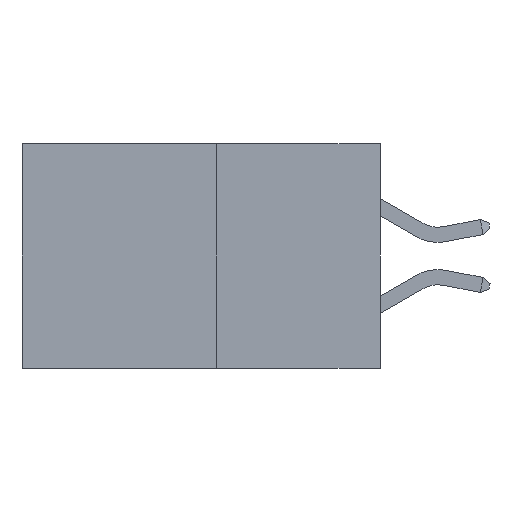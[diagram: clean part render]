
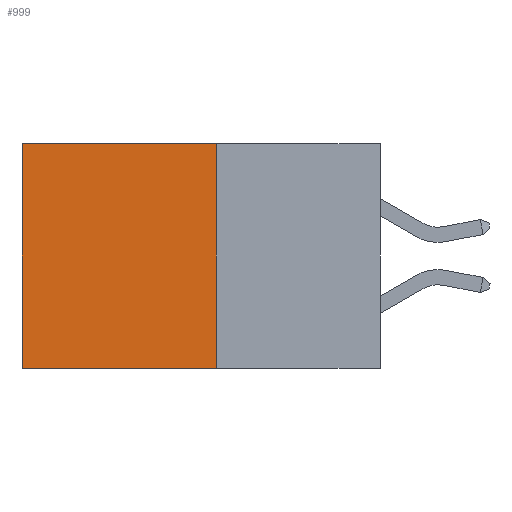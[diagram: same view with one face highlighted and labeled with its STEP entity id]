
A CAD part, left-side view. The second image highlights one B-rep face of the part: STEP entity #999.
In plain terms, the highlighted planar face has unit normal (-1, 0, 0).
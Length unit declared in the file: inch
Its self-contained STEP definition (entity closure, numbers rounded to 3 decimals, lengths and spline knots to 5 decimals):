
#92 = VERTEX_POINT ( 'NONE', #8112 ) ;
#236 = LINE ( 'NONE', #5766, #2025 ) ;
#418 = LINE ( 'NONE', #3237, #6210 ) ;
#638 = ORIENTED_EDGE ( 'NONE', *, *, #937, .F. ) ;
#935 = VECTOR ( 'NONE', #5083, 39.37008 ) ;
#937 = EDGE_CURVE ( 'NONE', #7355, #5221, #236, .T. ) ;
#999 = ADVANCED_FACE ( 'NONE', ( #5289 ), #2363, .F. ) ;
#2025 = VECTOR ( 'NONE', #2030, 39.37008 ) ;
#2030 = DIRECTION ( 'NONE',  ( 0., 0., -1. ) ) ;
#2363 = PLANE ( 'NONE',  #3022 ) ;
#2632 = ORIENTED_EDGE ( 'NONE', *, *, #5029, .T. ) ;
#3022 = AXIS2_PLACEMENT_3D ( 'NONE', #3222, #3078, #7476 ) ;
#3078 = DIRECTION ( 'NONE',  ( 1., 0., 0. ) ) ;
#3222 = CARTESIAN_POINT ( 'NONE',  ( 0.277, 0.27, -0.37 ) ) ;
#3237 = CARTESIAN_POINT ( 'NONE',  ( 0.277, 0.27, -0.37 ) ) ;
#3325 = EDGE_LOOP ( 'NONE', ( #6174, #8349, #638, #2632 ) ) ;
#3417 = EDGE_CURVE ( 'NONE', #5576, #92, #6691, .T. ) ;
#3563 = CARTESIAN_POINT ( 'NONE',  ( 0.277, 0.59, -0.37 ) ) ;
#3628 = CARTESIAN_POINT ( 'NONE',  ( 0.277, 0.27, -0.37 ) ) ;
#3979 = DIRECTION ( 'NONE',  ( 0., 1., 0. ) ) ;
#4792 = CARTESIAN_POINT ( 'NONE',  ( 0.277, 0.59, 0. ) ) ;
#5029 = EDGE_CURVE ( 'NONE', #7355, #5576, #6003, .T. ) ;
#5077 = CARTESIAN_POINT ( 'NONE',  ( 0.277, 0.27, 0. ) ) ;
#5083 = DIRECTION ( 'NONE',  ( 0., 0., -1. ) ) ;
#5221 = VERTEX_POINT ( 'NONE', #3628 ) ;
#5289 = FACE_OUTER_BOUND ( 'NONE', #3325, .T. ) ;
#5576 = VERTEX_POINT ( 'NONE', #4792 ) ;
#5596 = CARTESIAN_POINT ( 'NONE',  ( 0.277, 0.27, 0. ) ) ;
#5659 = DIRECTION ( 'NONE',  ( 0., 1., 0. ) ) ;
#5766 = CARTESIAN_POINT ( 'NONE',  ( 0.277, 0.27, -0.37 ) ) ;
#6003 = LINE ( 'NONE', #5596, #6242 ) ;
#6174 = ORIENTED_EDGE ( 'NONE', *, *, #3417, .T. ) ;
#6210 = VECTOR ( 'NONE', #3979, 39.37008 ) ;
#6242 = VECTOR ( 'NONE', #5659, 39.37008 ) ;
#6691 = LINE ( 'NONE', #3563, #935 ) ;
#7355 = VERTEX_POINT ( 'NONE', #5077 ) ;
#7476 = DIRECTION ( 'NONE',  ( 0., 0., -1. ) ) ;
#7712 = EDGE_CURVE ( 'NONE', #5221, #92, #418, .T. ) ;
#8112 = CARTESIAN_POINT ( 'NONE',  ( 0.277, 0.59, -0.37 ) ) ;
#8349 = ORIENTED_EDGE ( 'NONE', *, *, #7712, .F. ) ;
